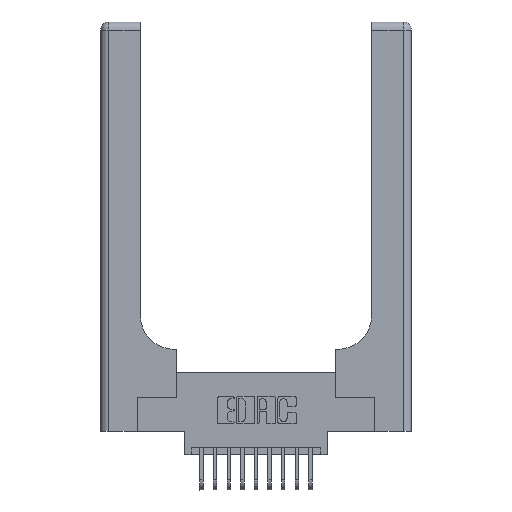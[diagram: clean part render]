
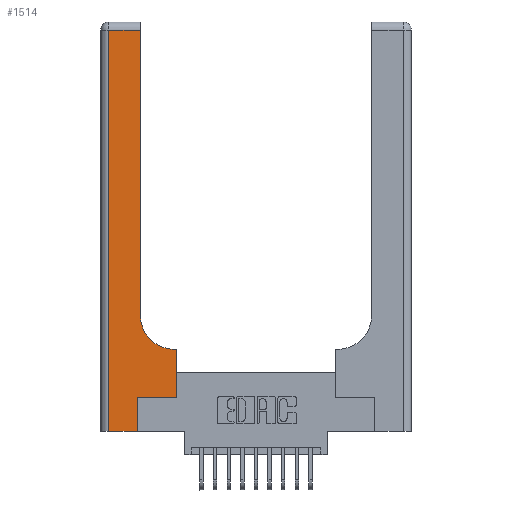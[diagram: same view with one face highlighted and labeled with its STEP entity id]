
A CAD part, top view. The second image highlights one B-rep face of the part: STEP entity #1514.
In plain terms, the highlighted planar face has unit normal (0, 0, 1).
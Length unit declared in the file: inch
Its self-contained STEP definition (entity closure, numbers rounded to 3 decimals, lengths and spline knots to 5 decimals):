
#496 = CARTESIAN_POINT ( 'NONE',  ( 0.2915, 0.85, 0.37 ) ) ;
#521 = CARTESIAN_POINT ( 'NONE',  ( 0.2915, 3., 0.37 ) ) ;
#653 = CARTESIAN_POINT ( 'NONE',  ( 0., 0., 0.37 ) ) ;
#949 = VERTEX_POINT ( 'NONE', #1041 ) ;
#1041 = CARTESIAN_POINT ( 'NONE',  ( 0.06, 0., 0.37 ) ) ;
#1080 = VERTEX_POINT ( 'NONE', #1276 ) ;
#1156 = EDGE_CURVE ( 'NONE', #15354, #949, #11711, .T. ) ;
#1276 = CARTESIAN_POINT ( 'NONE',  ( 0.269, 0., 0.37 ) ) ;
#1514 = ADVANCED_FACE ( 'NONE', ( #10310 ), #3764, .F. ) ;
#1516 = VERTEX_POINT ( 'NONE', #8860 ) ;
#1917 = EDGE_CURVE ( 'NONE', #949, #1080, #8894, .T. ) ;
#2055 = CARTESIAN_POINT ( 'NONE',  ( 0.2915, 0.6, 0.37 ) ) ;
#2431 = CARTESIAN_POINT ( 'NONE',  ( 0.5585, 0.25, 0.37 ) ) ;
#3019 = ORIENTED_EDGE ( 'NONE', *, *, #16031, .T. ) ;
#3390 = DIRECTION ( 'NONE',  ( -1., 0., 0. ) ) ;
#3740 = CARTESIAN_POINT ( 'NONE',  ( 0.5585, 0.25, 0.37 ) ) ;
#3764 = PLANE ( 'NONE',  #14182 ) ;
#3847 = CARTESIAN_POINT ( 'NONE',  ( 0.5415, 0.6, 0.37 ) ) ;
#3853 = LINE ( 'NONE', #5611, #9459 ) ;
#4145 = LINE ( 'NONE', #3740, #7189 ) ;
#4213 = CARTESIAN_POINT ( 'NONE',  ( 0.06, 3., 0.37 ) ) ;
#4400 = CARTESIAN_POINT ( 'NONE',  ( 0.2915, 2.94, 0.37 ) ) ;
#4947 = DIRECTION ( 'NONE',  ( -1., 0., 0. ) ) ;
#5053 = DIRECTION ( 'NONE',  ( -1., 0., 0. ) ) ;
#5611 = CARTESIAN_POINT ( 'NONE',  ( 0.269, 0., 0.37 ) ) ;
#5761 = CARTESIAN_POINT ( 'NONE',  ( 0.269, 0.25, 0.37 ) ) ;
#6029 = VERTEX_POINT ( 'NONE', #4400 ) ;
#6704 = CARTESIAN_POINT ( 'NONE',  ( 0.5415, 0.85, 0.37 ) ) ;
#6923 = DIRECTION ( 'NONE',  ( 0., 1., 0. ) ) ;
#6972 = VERTEX_POINT ( 'NONE', #496 ) ;
#7189 = VECTOR ( 'NONE', #13893, 39.37008 ) ;
#7282 = CARTESIAN_POINT ( 'NONE',  ( 0.5585, 0.6, 0.37 ) ) ;
#7918 = VECTOR ( 'NONE', #11881, 39.37008 ) ;
#7984 = DIRECTION ( 'NONE',  ( 1., 0., 0. ) ) ;
#8006 = EDGE_CURVE ( 'NONE', #9102, #6972, #13214, .T. ) ;
#8091 = VECTOR ( 'NONE', #11043, 39.37008 ) ;
#8349 = DIRECTION ( 'NONE',  ( 1., 0., 0. ) ) ;
#8507 = VERTEX_POINT ( 'NONE', #2431 ) ;
#8764 = EDGE_CURVE ( 'NONE', #1516, #8507, #12995, .T. ) ;
#8860 = CARTESIAN_POINT ( 'NONE',  ( 0.269, 0.25, 0.37 ) ) ;
#8894 = LINE ( 'NONE', #653, #8091 ) ;
#9102 = VERTEX_POINT ( 'NONE', #3847 ) ;
#9168 = LINE ( 'NONE', #2055, #15494 ) ;
#9459 = VECTOR ( 'NONE', #6923, 39.37008 ) ;
#9502 = AXIS2_PLACEMENT_3D ( 'NONE', #6704, #15555, #7984 ) ;
#9595 = DIRECTION ( 'NONE',  ( 0., 1., 0. ) ) ;
#10310 = FACE_OUTER_BOUND ( 'NONE', #14379, .T. ) ;
#10475 = ORIENTED_EDGE ( 'NONE', *, *, #10651, .T. ) ;
#10651 = EDGE_CURVE ( 'NONE', #14986, #9102, #9168, .T. ) ;
#10779 = EDGE_CURVE ( 'NONE', #8507, #14986, #4145, .T. ) ;
#10825 = ORIENTED_EDGE ( 'NONE', *, *, #15751, .T. ) ;
#11029 = ORIENTED_EDGE ( 'NONE', *, *, #1156, .T. ) ;
#11043 = DIRECTION ( 'NONE',  ( 1., 0., 0. ) ) ;
#11074 = ORIENTED_EDGE ( 'NONE', *, *, #8764, .T. ) ;
#11465 = ORIENTED_EDGE ( 'NONE', *, *, #15534, .T. ) ;
#11711 = LINE ( 'NONE', #4213, #7918 ) ;
#11822 = CARTESIAN_POINT ( 'NONE',  ( 0.06, 2.94, 0.37 ) ) ;
#11881 = DIRECTION ( 'NONE',  ( 0., -1., 0. ) ) ;
#12583 = CARTESIAN_POINT ( 'NONE',  ( 0., 2.94, 0.37 ) ) ;
#12703 = DIRECTION ( 'NONE',  ( 0., 0., -1. ) ) ;
#12859 = LINE ( 'NONE', #521, #16594 ) ;
#12995 = LINE ( 'NONE', #5761, #15549 ) ;
#13214 = CIRCLE ( 'NONE', #9502, 0.25 ) ;
#13893 = DIRECTION ( 'NONE',  ( 0., 1., 0. ) ) ;
#14182 = AXIS2_PLACEMENT_3D ( 'NONE', #16441, #12703, #5053 ) ;
#14229 = ORIENTED_EDGE ( 'NONE', *, *, #8006, .T. ) ;
#14379 = EDGE_LOOP ( 'NONE', ( #11465, #10825, #11029, #15770, #3019, #11074, #15980, #10475, #14229 ) ) ;
#14986 = VERTEX_POINT ( 'NONE', #7282 ) ;
#15354 = VERTEX_POINT ( 'NONE', #11822 ) ;
#15494 = VECTOR ( 'NONE', #3390, 39.37008 ) ;
#15534 = EDGE_CURVE ( 'NONE', #6972, #6029, #12859, .T. ) ;
#15549 = VECTOR ( 'NONE', #8349, 39.37008 ) ;
#15555 = DIRECTION ( 'NONE',  ( 0., 0., -1. ) ) ;
#15751 = EDGE_CURVE ( 'NONE', #6029, #15354, #16386, .T. ) ;
#15770 = ORIENTED_EDGE ( 'NONE', *, *, #1917, .T. ) ;
#15980 = ORIENTED_EDGE ( 'NONE', *, *, #10779, .T. ) ;
#15986 = VECTOR ( 'NONE', #4947, 39.37008 ) ;
#16031 = EDGE_CURVE ( 'NONE', #1080, #1516, #3853, .T. ) ;
#16386 = LINE ( 'NONE', #12583, #15986 ) ;
#16441 = CARTESIAN_POINT ( 'NONE',  ( 0., 3., 0.37 ) ) ;
#16594 = VECTOR ( 'NONE', #9595, 39.37008 ) ;
